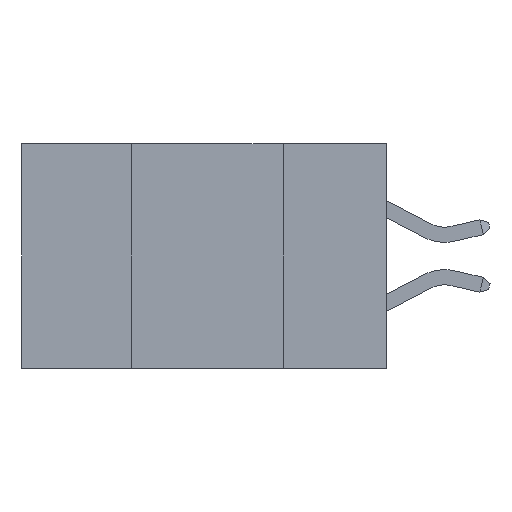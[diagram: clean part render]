
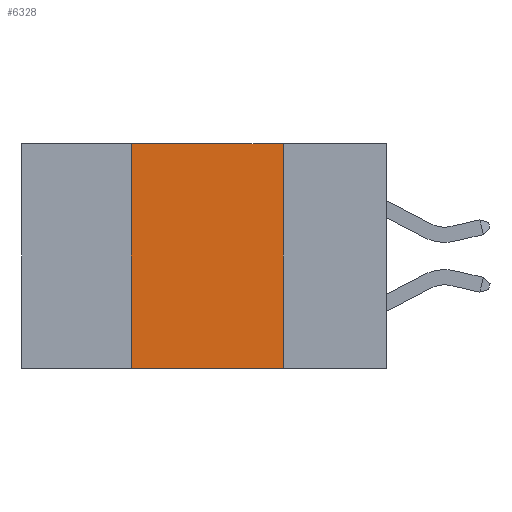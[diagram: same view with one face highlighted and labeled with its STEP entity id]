
A CAD part, left-side view. The second image highlights one B-rep face of the part: STEP entity #6328.
In plain terms, the highlighted planar face has unit normal (-1, 0, 0).
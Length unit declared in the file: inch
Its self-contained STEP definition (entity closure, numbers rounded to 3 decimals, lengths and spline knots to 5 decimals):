
#862 = VERTEX_POINT ( 'NONE', #16246 ) ;
#1204 = EDGE_CURVE ( 'NONE', #16494, #862, #15062, .T. ) ;
#1390 = ORIENTED_EDGE ( 'NONE', *, *, #12246, .F. ) ;
#3064 = DIRECTION ( 'NONE',  ( 0., 0., -1. ) ) ;
#4548 = CARTESIAN_POINT ( 'NONE',  ( 0., 0.6, 0. ) ) ;
#4759 = VECTOR ( 'NONE', #11503, 39.37008 ) ;
#5361 = AXIS2_PLACEMENT_3D ( 'NONE', #4548, #16377, #3064 ) ;
#6328 = ADVANCED_FACE ( 'NONE', ( #7196 ), #6421, .F. ) ;
#6421 = PLANE ( 'NONE',  #5361 ) ;
#6633 = LINE ( 'NONE', #18232, #4759 ) ;
#7196 = FACE_OUTER_BOUND ( 'NONE', #17035, .T. ) ;
#8184 = VERTEX_POINT ( 'NONE', #14042 ) ;
#8482 = EDGE_CURVE ( 'NONE', #16494, #8184, #17145, .T. ) ;
#8728 = ORIENTED_EDGE ( 'NONE', *, *, #8482, .T. ) ;
#10175 = LINE ( 'NONE', #11275, #14929 ) ;
#11275 = CARTESIAN_POINT ( 'NONE',  ( 0., 0.17, 0. ) ) ;
#11503 = DIRECTION ( 'NONE',  ( 0., -1., 0. ) ) ;
#12237 = ORIENTED_EDGE ( 'NONE', *, *, #15788, .F. ) ;
#12246 = EDGE_CURVE ( 'NONE', #17503, #8184, #10175, .T. ) ;
#12345 = DIRECTION ( 'NONE',  ( 0., 0., 1. ) ) ;
#12403 = CARTESIAN_POINT ( 'NONE',  ( 0., 0.17, 0. ) ) ;
#12832 = CARTESIAN_POINT ( 'NONE',  ( 0., 0.6, -0.37 ) ) ;
#14042 = CARTESIAN_POINT ( 'NONE',  ( 0., 0.17, -0.37 ) ) ;
#14274 = VECTOR ( 'NONE', #12345, 39.37008 ) ;
#14826 = ORIENTED_EDGE ( 'NONE', *, *, #1204, .F. ) ;
#14929 = VECTOR ( 'NONE', #18211, 39.37008 ) ;
#14968 = CARTESIAN_POINT ( 'NONE',  ( 0., 0.42, 0. ) ) ;
#15062 = LINE ( 'NONE', #14968, #14274 ) ;
#15788 = EDGE_CURVE ( 'NONE', #862, #17503, #6633, .T. ) ;
#16062 = VECTOR ( 'NONE', #19568, 39.37008 ) ;
#16246 = CARTESIAN_POINT ( 'NONE',  ( 0., 0.42, 0. ) ) ;
#16377 = DIRECTION ( 'NONE',  ( 1., 0., 0. ) ) ;
#16494 = VERTEX_POINT ( 'NONE', #18086 ) ;
#17035 = EDGE_LOOP ( 'NONE', ( #1390, #12237, #14826, #8728 ) ) ;
#17145 = LINE ( 'NONE', #12832, #16062 ) ;
#17503 = VERTEX_POINT ( 'NONE', #12403 ) ;
#18086 = CARTESIAN_POINT ( 'NONE',  ( 0., 0.42, -0.37 ) ) ;
#18211 = DIRECTION ( 'NONE',  ( 0., 0., -1. ) ) ;
#18232 = CARTESIAN_POINT ( 'NONE',  ( 0., 0.6, 0. ) ) ;
#19568 = DIRECTION ( 'NONE',  ( 0., -1., 0. ) ) ;
